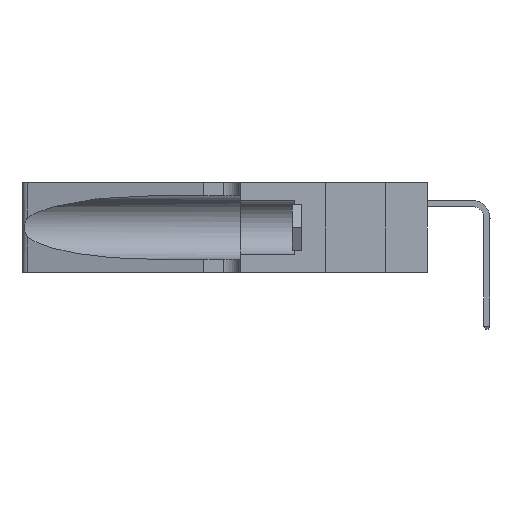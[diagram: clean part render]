
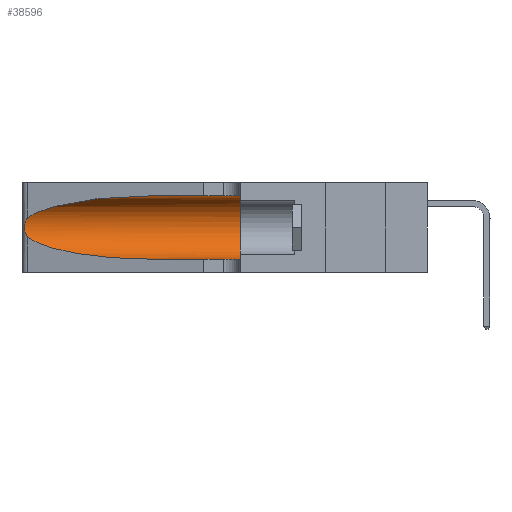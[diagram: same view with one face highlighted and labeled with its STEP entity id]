
A CAD part, left-side view. The second image highlights one B-rep face of the part: STEP entity #38596.
In plain terms, the highlighted cylindrical face has radius 3.308 mm (diameter 6.617 mm), a partial arc.
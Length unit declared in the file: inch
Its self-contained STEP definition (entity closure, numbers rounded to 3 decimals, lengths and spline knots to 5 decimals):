
#143 = CYLINDRICAL_SURFACE ( 'NONE', #9474, 0.13025 ) ;
#903 = DIRECTION ( 'NONE',  ( 0., 1., 0. ) ) ;
#1068 = ORIENTED_EDGE ( 'NONE', *, *, #24613, .T. ) ;
#1198 = FACE_OUTER_BOUND ( 'NONE', #39249, .T. ) ;
#1524 = CARTESIAN_POINT ( 'NONE',  ( 0.26075, 1.23896, 0.178 ) ) ;
#1671 = EDGE_CURVE ( 'NONE', #3960, #15132, #12854, .T. ) ;
#1727 = CARTESIAN_POINT ( 'NONE',  ( 0.1305, 1.61858, 0.05475 ) ) ;
#3960 = VERTEX_POINT ( 'NONE', #40261 ) ;
#4103 = CARTESIAN_POINT ( 'NONE',  ( 0.1305, 1.61858, 0.185 ) ) ;
#4961 = CARTESIAN_POINT ( 'NONE',  ( 0.25856, 1.23593, 0.16098 ) ) ;
#7498 = DIRECTION ( 'NONE',  ( 0., -1., 0. ) ) ;
#8343 = CARTESIAN_POINT ( 'NONE',  ( 0.25639, 1.23186, 0.15144 ) ) ;
#8603 = CARTESIAN_POINT ( 'NONE',  ( 0.1305, 0.72297, 0.31525 ) ) ;
#8806 = B_SPLINE_CURVE_WITH_KNOTS ( 'NONE', 3,
 ( #14872, #31519, #20855, #38190, #18252, #41513, #21590, #1524, #24940, #4961, #28321, #8343, #31664, #11674 ),
 .UNSPECIFIED., .F., .F.,
 ( 4, 2, 2, 2, 2, 2, 4 ),
 ( 0., 0.00027, 0.00053, 0.00107, 0.0016, 0.00187, 0.00214 ),
 .UNSPECIFIED. ) ;
#9308 = CARTESIAN_POINT ( 'NONE',  ( 0.1305, 0.72297, 0.31525 ) ) ;
#9474 = AXIS2_PLACEMENT_3D ( 'NONE', #4103, #7498, #20611 ) ;
#11674 = CARTESIAN_POINT ( 'NONE',  ( 0.25487, 1.22718, 0.14631 ) ) ;
#12290 = EDGE_CURVE ( 'NONE', #19521, #13214, #8806, .T. ) ;
#12854 = LINE ( 'NONE', #1727, #29603 ) ;
#13214 = VERTEX_POINT ( 'NONE', #19674 ) ;
#13321 =( BOUNDED_CURVE ( )  B_SPLINE_CURVE ( 3, ( #9308, #29294, #39313, #19360 ),
 .UNSPECIFIED., .F., .T. ) 
 B_SPLINE_CURVE_WITH_KNOTS ( ( 4, 4 ),
 ( 1.5708, 2.84003 ),
 .UNSPECIFIED. ) 
 CURVE ( )  GEOMETRIC_REPRESENTATION_ITEM ( )  RATIONAL_B_SPLINE_CURVE ( ( 1., 0.87, 0.87, 1. ) ) 
 REPRESENTATION_ITEM ( '' )  );
#14872 = CARTESIAN_POINT ( 'NONE',  ( 0.25487, 1.22718, 0.22369 ) ) ;
#15132 = VERTEX_POINT ( 'NONE', #23299 ) ;
#17464 = EDGE_CURVE ( 'NONE', #13214, #3960, #28863, .T. ) ;
#18252 = CARTESIAN_POINT ( 'NONE',  ( 0.25854, 1.2359, 0.20912 ) ) ;
#18307 = ORIENTED_EDGE ( 'NONE', *, *, #21613, .F. ) ;
#19360 = CARTESIAN_POINT ( 'NONE',  ( 0.25487, 1.22718, 0.22369 ) ) ;
#19521 = VERTEX_POINT ( 'NONE', #26995 ) ;
#19674 = CARTESIAN_POINT ( 'NONE',  ( 0.25487, 1.22718, 0.14631 ) ) ;
#19736 = CIRCLE ( 'NONE', #21650, 0.13025 ) ;
#20611 = DIRECTION ( 'NONE',  ( 0., 0., -1. ) ) ;
#20855 = CARTESIAN_POINT ( 'NONE',  ( 0.25639, 1.23184, 0.21858 ) ) ;
#20965 = CARTESIAN_POINT ( 'NONE',  ( 0.1305, 0.35, 0.185 ) ) ;
#21590 = CARTESIAN_POINT ( 'NONE',  ( 0.26075, 1.23896, 0.19203 ) ) ;
#21613 = EDGE_CURVE ( 'NONE', #32569, #15132, #19736, .T. ) ;
#21650 = AXIS2_PLACEMENT_3D ( 'NONE', #20965, #903, #24305 ) ;
#22606 = DIRECTION ( 'NONE',  ( 0., -1., 0. ) ) ;
#22781 = CARTESIAN_POINT ( 'NONE',  ( 0.2373, 1.15595, 0.08982 ) ) ;
#22929 = CARTESIAN_POINT ( 'NONE',  ( 0.1305, 0.72297, 0.05475 ) ) ;
#23299 = CARTESIAN_POINT ( 'NONE',  ( 0.1305, 0.35, 0.05475 ) ) ;
#24305 = DIRECTION ( 'NONE',  ( 0., 0., 1. ) ) ;
#24613 = EDGE_CURVE ( 'NONE', #37516, #19521, #13321, .T. ) ;
#24940 = CARTESIAN_POINT ( 'NONE',  ( 0.26017, 1.23833, 0.17102 ) ) ;
#26995 = CARTESIAN_POINT ( 'NONE',  ( 0.25487, 1.22718, 0.22369 ) ) ;
#27105 = CARTESIAN_POINT ( 'NONE',  ( 0.1305, 0.35, 0.31525 ) ) ;
#27834 = ORIENTED_EDGE ( 'NONE', *, *, #12290, .T. ) ;
#28321 = CARTESIAN_POINT ( 'NONE',  ( 0.25789, 1.23486, 0.15765 ) ) ;
#28863 =( BOUNDED_CURVE ( )  B_SPLINE_CURVE ( 3, ( #36148, #22781, #42832, #22929 ),
 .UNSPECIFIED., .F., .T. ) 
 B_SPLINE_CURVE_WITH_KNOTS ( ( 4, 4 ),
 ( 3.44316, 4.71239 ),
 .UNSPECIFIED. ) 
 CURVE ( )  GEOMETRIC_REPRESENTATION_ITEM ( )  RATIONAL_B_SPLINE_CURVE ( ( 1., 0.87, 0.87, 1. ) ) 
 REPRESENTATION_ITEM ( '' )  );
#29294 = CARTESIAN_POINT ( 'NONE',  ( 0.18966, 0.96281, 0.31525 ) ) ;
#29397 = VECTOR ( 'NONE', #22606, 39.37008 ) ;
#29603 = VECTOR ( 'NONE', #41701, 39.37008 ) ;
#30432 = LINE ( 'NONE', #35832, #29397 ) ;
#31519 = CARTESIAN_POINT ( 'NONE',  ( 0.25555, 1.22994, 0.2215 ) ) ;
#31664 = CARTESIAN_POINT ( 'NONE',  ( 0.25555, 1.22993, 0.14849 ) ) ;
#32146 = ORIENTED_EDGE ( 'NONE', *, *, #39569, .F. ) ;
#32569 = VERTEX_POINT ( 'NONE', #27105 ) ;
#35832 = CARTESIAN_POINT ( 'NONE',  ( 0.1305, 1.61858, 0.31525 ) ) ;
#36148 = CARTESIAN_POINT ( 'NONE',  ( 0.25487, 1.22718, 0.14631 ) ) ;
#37516 = VERTEX_POINT ( 'NONE', #8603 ) ;
#38190 = CARTESIAN_POINT ( 'NONE',  ( 0.25787, 1.23484, 0.2124 ) ) ;
#38345 = ORIENTED_EDGE ( 'NONE', *, *, #1671, .T. ) ;
#38596 = ADVANCED_FACE ( 'NONE', ( #1198 ), #143, .F. ) ;
#39249 = EDGE_LOOP ( 'NONE', ( #1068, #27834, #42621, #38345, #18307, #32146 ) ) ;
#39313 = CARTESIAN_POINT ( 'NONE',  ( 0.2373, 1.15595, 0.28018 ) ) ;
#39569 = EDGE_CURVE ( 'NONE', #37516, #32569, #30432, .T. ) ;
#40261 = CARTESIAN_POINT ( 'NONE',  ( 0.1305, 0.72297, 0.05475 ) ) ;
#41513 = CARTESIAN_POINT ( 'NONE',  ( 0.26018, 1.23835, 0.19895 ) ) ;
#41701 = DIRECTION ( 'NONE',  ( 0., -1., 0. ) ) ;
#42621 = ORIENTED_EDGE ( 'NONE', *, *, #17464, .T. ) ;
#42832 = CARTESIAN_POINT ( 'NONE',  ( 0.18966, 0.96281, 0.05475 ) ) ;
